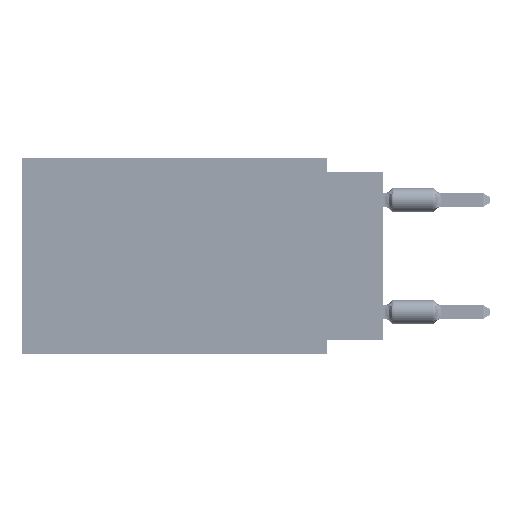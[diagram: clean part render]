
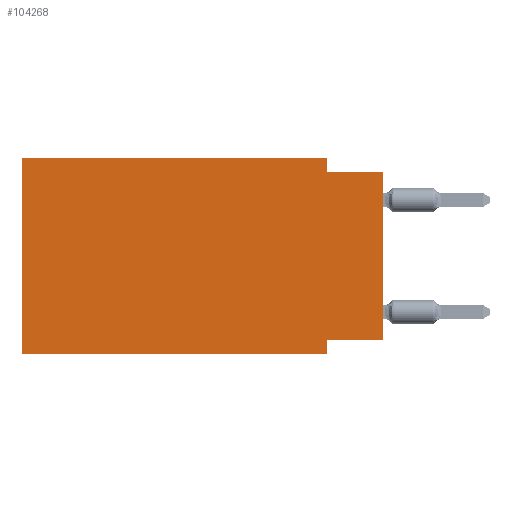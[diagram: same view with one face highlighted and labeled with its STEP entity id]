
A CAD part, left-side view. The second image highlights one B-rep face of the part: STEP entity #104268.
In plain terms, the highlighted planar face has unit normal (-1, 0, 0).
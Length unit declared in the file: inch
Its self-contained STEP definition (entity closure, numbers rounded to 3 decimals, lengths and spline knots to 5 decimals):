
#111 = CARTESIAN_POINT ( 'NONE',  ( 0., 0.1, -0.025 ) ) ;
#176 = CARTESIAN_POINT ( 'NONE',  ( 0., 0.645, 0. ) ) ;
#1116 = DIRECTION ( 'NONE',  ( 0., 0., -1. ) ) ;
#1758 = VERTEX_POINT ( 'NONE', #81151 ) ;
#6360 = VECTOR ( 'NONE', #7480, 39.37008 ) ;
#6770 = EDGE_CURVE ( 'NONE', #15526, #104943, #43298, .T. ) ;
#7480 = DIRECTION ( 'NONE',  ( 0., 0., 1. ) ) ;
#8705 = LINE ( 'NONE', #117381, #71079 ) ;
#11059 = ORIENTED_EDGE ( 'NONE', *, *, #107237, .F. ) ;
#13468 = DIRECTION ( 'NONE',  ( 0., -1., 0. ) ) ;
#15194 = EDGE_CURVE ( 'NONE', #85569, #1758, #107369, .T. ) ;
#15526 = VERTEX_POINT ( 'NONE', #17702 ) ;
#16482 = CARTESIAN_POINT ( 'NONE',  ( 0., 0.645, 0. ) ) ;
#17702 = CARTESIAN_POINT ( 'NONE',  ( 0., 0.645, 0. ) ) ;
#23548 = VERTEX_POINT ( 'NONE', #107679 ) ;
#26589 = PLANE ( 'NONE',  #103125 ) ;
#27034 = CARTESIAN_POINT ( 'NONE',  ( 0., 0.645, 0. ) ) ;
#30107 = EDGE_CURVE ( 'NONE', #23548, #59428, #105481, .T. ) ;
#32058 = VECTOR ( 'NONE', #89516, 39.37008 ) ;
#32419 = VECTOR ( 'NONE', #117543, 39.37008 ) ;
#33543 = LINE ( 'NONE', #53319, #32419 ) ;
#35192 = CARTESIAN_POINT ( 'NONE',  ( 0., 0.645, -0.35 ) ) ;
#38124 = EDGE_CURVE ( 'NONE', #110637, #59428, #49492, .T. ) ;
#41093 = VERTEX_POINT ( 'NONE', #35192 ) ;
#43298 = LINE ( 'NONE', #27034, #32058 ) ;
#45803 = FACE_OUTER_BOUND ( 'NONE', #72723, .T. ) ;
#49492 = LINE ( 'NONE', #69271, #115024 ) ;
#50469 = ORIENTED_EDGE ( 'NONE', *, *, #30107, .T. ) ;
#53319 = CARTESIAN_POINT ( 'NONE',  ( 0., 0., -0.325 ) ) ;
#53427 = ORIENTED_EDGE ( 'NONE', *, *, #78102, .T. ) ;
#57541 = LINE ( 'NONE', #65953, #85773 ) ;
#59428 = VERTEX_POINT ( 'NONE', #115506 ) ;
#61748 = DIRECTION ( 'NONE',  ( 0., 0., -1. ) ) ;
#61789 = EDGE_CURVE ( 'NONE', #104943, #110637, #57541, .T. ) ;
#63217 = DIRECTION ( 'NONE',  ( 1., 0., 0. ) ) ;
#65953 = CARTESIAN_POINT ( 'NONE',  ( 0., 0.1, 0. ) ) ;
#66857 = ORIENTED_EDGE ( 'NONE', *, *, #111954, .F. ) ;
#69271 = CARTESIAN_POINT ( 'NONE',  ( 0., 0., -0.025 ) ) ;
#71079 = VECTOR ( 'NONE', #72938, 39.37008 ) ;
#72723 = EDGE_LOOP ( 'NONE', ( #50469, #116698, #82981, #79298, #66857, #53427, #105955, #11059 ) ) ;
#72938 = DIRECTION ( 'NONE',  ( 0., -1., 0. ) ) ;
#78102 = EDGE_CURVE ( 'NONE', #41093, #1758, #8705, .T. ) ;
#79298 = ORIENTED_EDGE ( 'NONE', *, *, #6770, .F. ) ;
#79633 = CARTESIAN_POINT ( 'NONE',  ( 0., 0., 0. ) ) ;
#81151 = CARTESIAN_POINT ( 'NONE',  ( 0., 0.1, -0.35 ) ) ;
#82413 = DIRECTION ( 'NONE',  ( 0., 0., -1. ) ) ;
#82981 = ORIENTED_EDGE ( 'NONE', *, *, #61789, .F. ) ;
#85569 = VERTEX_POINT ( 'NONE', #87231 ) ;
#85773 = VECTOR ( 'NONE', #1116, 39.37008 ) ;
#87231 = CARTESIAN_POINT ( 'NONE',  ( 0., 0.1, -0.325 ) ) ;
#89516 = DIRECTION ( 'NONE',  ( 0., -1., 0. ) ) ;
#96004 = CARTESIAN_POINT ( 'NONE',  ( 0., 0.1, -0.35 ) ) ;
#102674 = VECTOR ( 'NONE', #61748, 39.37008 ) ;
#103125 = AXIS2_PLACEMENT_3D ( 'NONE', #176, #63217, #82413 ) ;
#104268 = ADVANCED_FACE ( 'NONE', ( #45803 ), #26589, .F. ) ;
#104943 = VERTEX_POINT ( 'NONE', #108391 ) ;
#105481 = LINE ( 'NONE', #79633, #108659 ) ;
#105955 = ORIENTED_EDGE ( 'NONE', *, *, #15194, .F. ) ;
#107237 = EDGE_CURVE ( 'NONE', #23548, #85569, #33543, .T. ) ;
#107369 = LINE ( 'NONE', #96004, #102674 ) ;
#107679 = CARTESIAN_POINT ( 'NONE',  ( 0., 0., -0.325 ) ) ;
#107737 = LINE ( 'NONE', #16482, #6360 ) ;
#108391 = CARTESIAN_POINT ( 'NONE',  ( 0., 0.1, 0. ) ) ;
#108659 = VECTOR ( 'NONE', #113891, 39.37008 ) ;
#110637 = VERTEX_POINT ( 'NONE', #111 ) ;
#111954 = EDGE_CURVE ( 'NONE', #41093, #15526, #107737, .T. ) ;
#113891 = DIRECTION ( 'NONE',  ( 0., 0., 1. ) ) ;
#115024 = VECTOR ( 'NONE', #13468, 39.37008 ) ;
#115506 = CARTESIAN_POINT ( 'NONE',  ( 0., 0., -0.025 ) ) ;
#116698 = ORIENTED_EDGE ( 'NONE', *, *, #38124, .F. ) ;
#117381 = CARTESIAN_POINT ( 'NONE',  ( 0., 0.645, -0.35 ) ) ;
#117543 = DIRECTION ( 'NONE',  ( 0., 1., 0. ) ) ;
